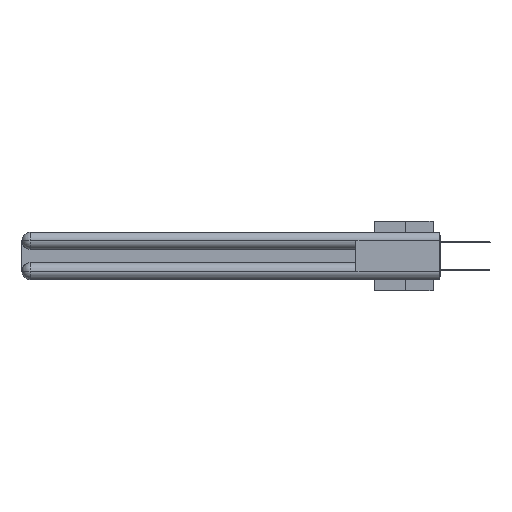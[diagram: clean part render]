
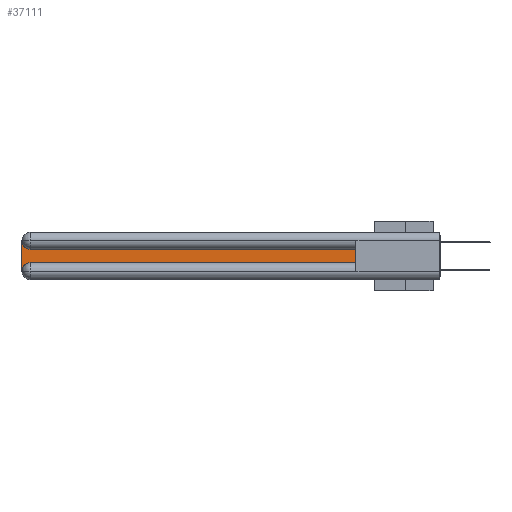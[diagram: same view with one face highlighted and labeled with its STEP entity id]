
A CAD part, left-side view. The second image highlights one B-rep face of the part: STEP entity #37111.
In plain terms, the highlighted planar face has unit normal (-1, 0, 0).
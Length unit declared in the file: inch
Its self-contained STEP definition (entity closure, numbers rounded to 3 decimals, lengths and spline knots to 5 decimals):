
#1451 = CARTESIAN_POINT ( 'NONE',  ( 0.075, 3., -0.2775 ) ) ;
#2863 = VECTOR ( 'NONE', #9902, 39.37008 ) ;
#3803 = DIRECTION ( 'NONE',  ( 0., 1., 0. ) ) ;
#4223 = DIRECTION ( 'NONE',  ( 1., 0., 0. ) ) ;
#4464 = EDGE_CURVE ( 'NONE', #29139, #4792, #16617, .T. ) ;
#4486 = VECTOR ( 'NONE', #31662, 39.37008 ) ;
#4792 = VERTEX_POINT ( 'NONE', #27661 ) ;
#4889 = DIRECTION ( 'NONE',  ( 0., 0., -1. ) ) ;
#5163 = VERTEX_POINT ( 'NONE', #31262 ) ;
#6681 = EDGE_CURVE ( 'NONE', #13817, #5163, #13237, .T. ) ;
#6778 = CARTESIAN_POINT ( 'NONE',  ( 0.075, 2.94, -0.2175 ) ) ;
#7957 = CARTESIAN_POINT ( 'NONE',  ( 0.075, 0.6, -0.2175 ) ) ;
#7961 = PLANE ( 'NONE',  #38940 ) ;
#8748 = DIRECTION ( 'NONE',  ( 0., 0., -1. ) ) ;
#9902 = DIRECTION ( 'NONE',  ( 0., -1., 0. ) ) ;
#10398 = CARTESIAN_POINT ( 'NONE',  ( 0.075, 0.6, -0.2175 ) ) ;
#10439 = CARTESIAN_POINT ( 'NONE',  ( 0.075, 2.94, -0.2775 ) ) ;
#11210 = FACE_OUTER_BOUND ( 'NONE', #11990, .T. ) ;
#11990 = EDGE_LOOP ( 'NONE', ( #34419, #29703, #27765, #29284, #15598, #23145 ) ) ;
#12646 = EDGE_CURVE ( 'NONE', #26812, #13817, #18068, .T. ) ;
#13237 = LINE ( 'NONE', #10398, #4486 ) ;
#13817 = VERTEX_POINT ( 'NONE', #7957 ) ;
#13911 = CARTESIAN_POINT ( 'NONE',  ( 0.075, 2.94, -0.0625 ) ) ;
#14356 = EDGE_CURVE ( 'NONE', #4792, #22568, #32634, .T. ) ;
#15598 = ORIENTED_EDGE ( 'NONE', *, *, #12646, .T. ) ;
#16617 = CIRCLE ( 'NONE', #28266, 0.06 ) ;
#16674 = EDGE_CURVE ( 'NONE', #5163, #29139, #24454, .T. ) ;
#16819 = CARTESIAN_POINT ( 'NONE',  ( 0.075, 3., -0.2175 ) ) ;
#18068 = LINE ( 'NONE', #33272, #2863 ) ;
#18705 = CIRCLE ( 'NONE', #24552, 0.06 ) ;
#20544 = DIRECTION ( 'NONE',  ( 1., 0., 0. ) ) ;
#22568 = VERTEX_POINT ( 'NONE', #1451 ) ;
#23145 = ORIENTED_EDGE ( 'NONE', *, *, #6681, .T. ) ;
#23556 = CARTESIAN_POINT ( 'NONE',  ( 0.075, 3., -0.1225 ) ) ;
#24088 = VECTOR ( 'NONE', #3803, 39.37008 ) ;
#24454 = LINE ( 'NONE', #36828, #24088 ) ;
#24552 = AXIS2_PLACEMENT_3D ( 'NONE', #10439, #20544, #32516 ) ;
#26712 = VECTOR ( 'NONE', #4889, 39.37008 ) ;
#26812 = VERTEX_POINT ( 'NONE', #6778 ) ;
#26852 = CARTESIAN_POINT ( 'NONE',  ( 0.075, 2.94, -0.1225 ) ) ;
#27661 = CARTESIAN_POINT ( 'NONE',  ( 0.075, 3., -0.0625 ) ) ;
#27765 = ORIENTED_EDGE ( 'NONE', *, *, #14356, .T. ) ;
#28266 = AXIS2_PLACEMENT_3D ( 'NONE', #13911, #4223, #37834 ) ;
#29139 = VERTEX_POINT ( 'NONE', #26852 ) ;
#29284 = ORIENTED_EDGE ( 'NONE', *, *, #32878, .T. ) ;
#29703 = ORIENTED_EDGE ( 'NONE', *, *, #4464, .T. ) ;
#31262 = CARTESIAN_POINT ( 'NONE',  ( 0.075, 0.6, -0.1225 ) ) ;
#31662 = DIRECTION ( 'NONE',  ( 0., 0., 1. ) ) ;
#32516 = DIRECTION ( 'NONE',  ( 0., 0., -1. ) ) ;
#32634 = LINE ( 'NONE', #16819, #26712 ) ;
#32878 = EDGE_CURVE ( 'NONE', #22568, #26812, #18705, .T. ) ;
#33272 = CARTESIAN_POINT ( 'NONE',  ( 0.075, 0.6, -0.2175 ) ) ;
#34419 = ORIENTED_EDGE ( 'NONE', *, *, #16674, .T. ) ;
#36536 = DIRECTION ( 'NONE',  ( 1., 0., 0. ) ) ;
#36828 = CARTESIAN_POINT ( 'NONE',  ( 0.075, 0.6, -0.1225 ) ) ;
#37111 = ADVANCED_FACE ( 'NONE', ( #11210 ), #7961, .F. ) ;
#37834 = DIRECTION ( 'NONE',  ( 0., 0., -1. ) ) ;
#38940 = AXIS2_PLACEMENT_3D ( 'NONE', #23556, #36536, #8748 ) ;
